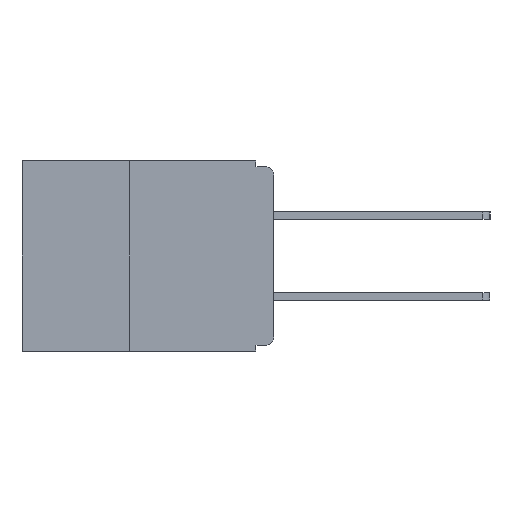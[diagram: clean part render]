
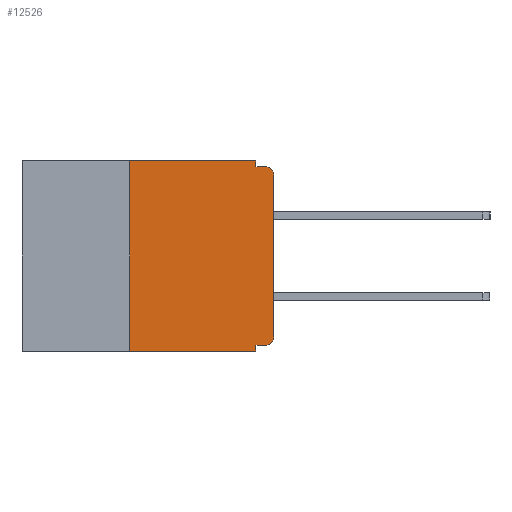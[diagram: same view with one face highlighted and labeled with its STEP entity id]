
A CAD part, left-side view. The second image highlights one B-rep face of the part: STEP entity #12526.
In plain terms, the highlighted planar face has unit normal (-1, 0, 0).
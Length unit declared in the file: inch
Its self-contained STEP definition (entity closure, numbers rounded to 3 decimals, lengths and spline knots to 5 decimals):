
#119 = VERTEX_POINT ( 'NONE', #14186 ) ;
#162 = DIRECTION ( 'NONE',  ( 0., 0., 1. ) ) ;
#389 = PLANE ( 'NONE',  #987 ) ;
#599 = EDGE_CURVE ( 'NONE', #119, #14799, #1966, .T. ) ;
#785 = ORIENTED_EDGE ( 'NONE', *, *, #6051, .T. ) ;
#953 = VERTEX_POINT ( 'NONE', #12132 ) ;
#971 = LINE ( 'NONE', #9310, #3170 ) ;
#987 = AXIS2_PLACEMENT_3D ( 'NONE', #5530, #9410, #1730 ) ;
#988 = CARTESIAN_POINT ( 'NONE',  ( 0., 0.031, 0. ) ) ;
#1730 = DIRECTION ( 'NONE',  ( 0., 0., -1. ) ) ;
#1739 = CARTESIAN_POINT ( 'NONE',  ( 0., 0., -0.305 ) ) ;
#1762 = VECTOR ( 'NONE', #3561, 39.37008 ) ;
#1966 = CIRCLE ( 'NONE', #9056, 0.015 ) ;
#2309 = VECTOR ( 'NONE', #162, 39.37008 ) ;
#2792 = ORIENTED_EDGE ( 'NONE', *, *, #599, .T. ) ;
#2970 = VECTOR ( 'NONE', #10986, 39.37008 ) ;
#3056 = VECTOR ( 'NONE', #10255, 39.37008 ) ;
#3170 = VECTOR ( 'NONE', #14298, 39.37008 ) ;
#3263 = CARTESIAN_POINT ( 'NONE',  ( 0., 0.25, 0. ) ) ;
#3270 = CARTESIAN_POINT ( 'NONE',  ( 0., 0., -0.01 ) ) ;
#3404 = EDGE_CURVE ( 'NONE', #953, #10873, #4269, .T. ) ;
#3561 = DIRECTION ( 'NONE',  ( 0., 0., -1. ) ) ;
#3679 = ORIENTED_EDGE ( 'NONE', *, *, #9942, .T. ) ;
#3685 = CARTESIAN_POINT ( 'NONE',  ( 0., 0.015, -0.025 ) ) ;
#3747 = EDGE_CURVE ( 'NONE', #9848, #14830, #12319, .T. ) ;
#3750 = LINE ( 'NONE', #3270, #2970 ) ;
#3787 = DIRECTION ( 'NONE',  ( 0., 0., -1. ) ) ;
#3893 = DIRECTION ( 'NONE',  ( -1., 0., 0. ) ) ;
#4269 = LINE ( 'NONE', #15190, #10721 ) ;
#4495 = CARTESIAN_POINT ( 'NONE',  ( 0., 0.031, -0.33 ) ) ;
#4750 = VERTEX_POINT ( 'NONE', #13742 ) ;
#4850 = ORIENTED_EDGE ( 'NONE', *, *, #13477, .F. ) ;
#5530 = CARTESIAN_POINT ( 'NONE',  ( 0., 0.437, 0. ) ) ;
#5826 = LINE ( 'NONE', #12405, #8837 ) ;
#5857 = ORIENTED_EDGE ( 'NONE', *, *, #10159, .F. ) ;
#5935 = FACE_OUTER_BOUND ( 'NONE', #13868, .T. ) ;
#6051 = EDGE_CURVE ( 'NONE', #14830, #119, #5826, .T. ) ;
#6375 = CARTESIAN_POINT ( 'NONE',  ( 0., 0.031, 0. ) ) ;
#6476 = LINE ( 'NONE', #16467, #3056 ) ;
#6713 = ORIENTED_EDGE ( 'NONE', *, *, #3404, .F. ) ;
#7054 = EDGE_CURVE ( 'NONE', #10903, #10518, #7812, .T. ) ;
#7812 = LINE ( 'NONE', #15826, #10820 ) ;
#7872 = EDGE_CURVE ( 'NONE', #10518, #4750, #8608, .T. ) ;
#8491 = ORIENTED_EDGE ( 'NONE', *, *, #7872, .F. ) ;
#8608 = LINE ( 'NONE', #988, #1762 ) ;
#8837 = VECTOR ( 'NONE', #11195, 39.37008 ) ;
#8971 = DIRECTION ( 'NONE',  ( 0., 0., -1. ) ) ;
#8975 = AXIS2_PLACEMENT_3D ( 'NONE', #9027, #9021, #8971 ) ;
#9021 = DIRECTION ( 'NONE',  ( -1., 0., 0. ) ) ;
#9027 = CARTESIAN_POINT ( 'NONE',  ( 0., 0.015, -0.305 ) ) ;
#9056 = AXIS2_PLACEMENT_3D ( 'NONE', #3685, #3893, #3787 ) ;
#9091 = CARTESIAN_POINT ( 'NONE',  ( 0., 0.015, -0.32 ) ) ;
#9129 = LINE ( 'NONE', #11781, #2309 ) ;
#9310 = CARTESIAN_POINT ( 'NONE',  ( 0., 0.437, -0.33 ) ) ;
#9410 = DIRECTION ( 'NONE',  ( 1., 0., 0. ) ) ;
#9848 = VERTEX_POINT ( 'NONE', #9091 ) ;
#9942 = EDGE_CURVE ( 'NONE', #11459, #10873, #971, .T. ) ;
#10159 = EDGE_CURVE ( 'NONE', #4750, #14799, #3750, .T. ) ;
#10255 = DIRECTION ( 'NONE',  ( 0., 1., 0. ) ) ;
#10518 = VERTEX_POINT ( 'NONE', #6375 ) ;
#10721 = VECTOR ( 'NONE', #15060, 39.37008 ) ;
#10820 = VECTOR ( 'NONE', #10860, 39.37008 ) ;
#10860 = DIRECTION ( 'NONE',  ( 0., -1., 0. ) ) ;
#10873 = VERTEX_POINT ( 'NONE', #4495 ) ;
#10903 = VERTEX_POINT ( 'NONE', #3263 ) ;
#10986 = DIRECTION ( 'NONE',  ( 0., -1., 0. ) ) ;
#11195 = DIRECTION ( 'NONE',  ( 0., 0., 1. ) ) ;
#11459 = VERTEX_POINT ( 'NONE', #12083 ) ;
#11781 = CARTESIAN_POINT ( 'NONE',  ( 0., 0.25, -0.33 ) ) ;
#11870 = ORIENTED_EDGE ( 'NONE', *, *, #3747, .T. ) ;
#12083 = CARTESIAN_POINT ( 'NONE',  ( 0., 0.25, -0.33 ) ) ;
#12132 = CARTESIAN_POINT ( 'NONE',  ( 0., 0.031, -0.32 ) ) ;
#12263 = ORIENTED_EDGE ( 'NONE', *, *, #15392, .F. ) ;
#12319 = CIRCLE ( 'NONE', #8975, 0.015 ) ;
#12405 = CARTESIAN_POINT ( 'NONE',  ( 0., 0., 0. ) ) ;
#12526 = ADVANCED_FACE ( 'NONE', ( #5935 ), #389, .F. ) ;
#13162 = CARTESIAN_POINT ( 'NONE',  ( 0., 0.015, -0.01 ) ) ;
#13477 = EDGE_CURVE ( 'NONE', #9848, #953, #6476, .T. ) ;
#13742 = CARTESIAN_POINT ( 'NONE',  ( 0., 0.031, -0.01 ) ) ;
#13868 = EDGE_LOOP ( 'NONE', ( #785, #2792, #5857, #8491, #14001, #12263, #3679, #6713, #4850, #11870 ) ) ;
#14001 = ORIENTED_EDGE ( 'NONE', *, *, #7054, .F. ) ;
#14186 = CARTESIAN_POINT ( 'NONE',  ( 0., 0., -0.025 ) ) ;
#14298 = DIRECTION ( 'NONE',  ( 0., -1., 0. ) ) ;
#14799 = VERTEX_POINT ( 'NONE', #13162 ) ;
#14830 = VERTEX_POINT ( 'NONE', #1739 ) ;
#15060 = DIRECTION ( 'NONE',  ( 0., 0., -1. ) ) ;
#15190 = CARTESIAN_POINT ( 'NONE',  ( 0., 0.031, -0.33 ) ) ;
#15392 = EDGE_CURVE ( 'NONE', #11459, #10903, #9129, .T. ) ;
#15826 = CARTESIAN_POINT ( 'NONE',  ( 0., 0.437, 0. ) ) ;
#16467 = CARTESIAN_POINT ( 'NONE',  ( 0., 0., -0.32 ) ) ;
